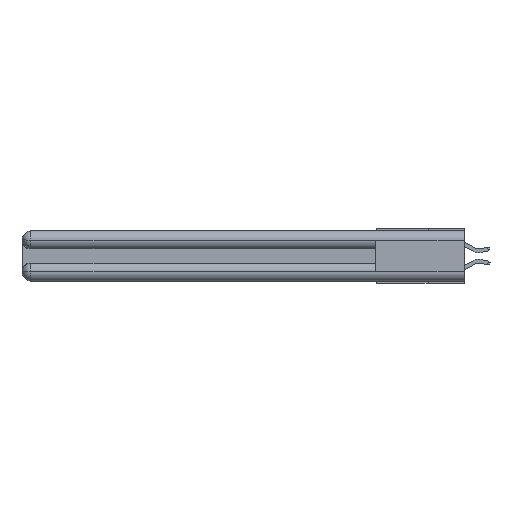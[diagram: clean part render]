
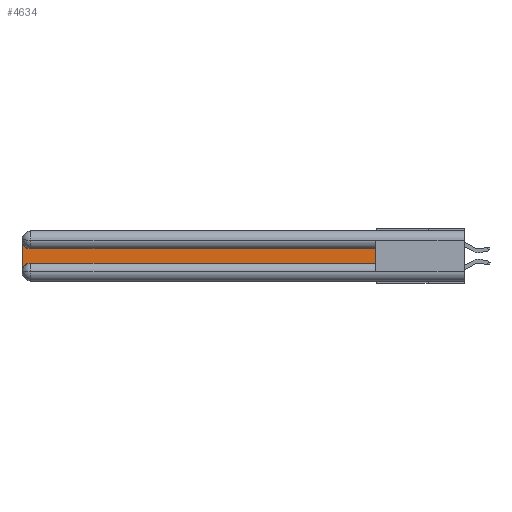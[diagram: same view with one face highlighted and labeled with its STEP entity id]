
A CAD part, left-side view. The second image highlights one B-rep face of the part: STEP entity #4634.
In plain terms, the highlighted planar face has unit normal (-1, 0, 0).
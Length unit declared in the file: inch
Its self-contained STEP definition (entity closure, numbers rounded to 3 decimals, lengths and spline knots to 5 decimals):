
#515 = VERTEX_POINT ( 'NONE', #25482 ) ;
#589 = CARTESIAN_POINT ( 'NONE',  ( 0.075, 2.94, -0.0625 ) ) ;
#709 = DIRECTION ( 'NONE',  ( 0., 0., -1. ) ) ;
#936 = DIRECTION ( 'NONE',  ( 1., 0., 0. ) ) ;
#1106 = LINE ( 'NONE', #28609, #12428 ) ;
#1406 = EDGE_CURVE ( 'NONE', #9785, #18341, #14608, .T. ) ;
#1716 = LINE ( 'NONE', #6207, #13897 ) ;
#3504 = CARTESIAN_POINT ( 'NONE',  ( 0.075, 3., -0.1225 ) ) ;
#4245 = VECTOR ( 'NONE', #32320, 39.37008 ) ;
#4634 = ADVANCED_FACE ( 'NONE', ( #17571 ), #8517, .F. ) ;
#5281 = CARTESIAN_POINT ( 'NONE',  ( 0.075, 2.94, -0.2775 ) ) ;
#5322 = EDGE_CURVE ( 'NONE', #18341, #7015, #23565, .T. ) ;
#6207 = CARTESIAN_POINT ( 'NONE',  ( 0.075, 0.6, -0.2175 ) ) ;
#7015 = VERTEX_POINT ( 'NONE', #17842 ) ;
#7834 = EDGE_CURVE ( 'NONE', #515, #26210, #1716, .T. ) ;
#8028 = LINE ( 'NONE', #23870, #4245 ) ;
#8517 = PLANE ( 'NONE',  #11452 ) ;
#9201 = CARTESIAN_POINT ( 'NONE',  ( 0.075, 0.6, -0.2175 ) ) ;
#9785 = VERTEX_POINT ( 'NONE', #31864 ) ;
#10254 = ORIENTED_EDGE ( 'NONE', *, *, #11381, .T. ) ;
#10398 = DIRECTION ( 'NONE',  ( 0., 0., -1. ) ) ;
#11381 = EDGE_CURVE ( 'NONE', #7015, #515, #17368, .T. ) ;
#11452 = AXIS2_PLACEMENT_3D ( 'NONE', #3504, #936, #27818 ) ;
#11609 = AXIS2_PLACEMENT_3D ( 'NONE', #589, #32872, #709 ) ;
#12428 = VECTOR ( 'NONE', #12513, 39.37008 ) ;
#12513 = DIRECTION ( 'NONE',  ( 0., 0., 1. ) ) ;
#13598 = ORIENTED_EDGE ( 'NONE', *, *, #15460, .T. ) ;
#13897 = VECTOR ( 'NONE', #33085, 39.37008 ) ;
#14351 = AXIS2_PLACEMENT_3D ( 'NONE', #5281, #26530, #10398 ) ;
#14608 = CIRCLE ( 'NONE', #11609, 0.06 ) ;
#14615 = DIRECTION ( 'NONE',  ( 0., 0., -1. ) ) ;
#15460 = EDGE_CURVE ( 'NONE', #26210, #25555, #1106, .T. ) ;
#17368 = CIRCLE ( 'NONE', #14351, 0.06 ) ;
#17571 = FACE_OUTER_BOUND ( 'NONE', #31752, .T. ) ;
#17842 = CARTESIAN_POINT ( 'NONE',  ( 0.075, 3., -0.2775 ) ) ;
#18116 = ORIENTED_EDGE ( 'NONE', *, *, #1406, .T. ) ;
#18341 = VERTEX_POINT ( 'NONE', #26505 ) ;
#19365 = ORIENTED_EDGE ( 'NONE', *, *, #7834, .T. ) ;
#19434 = ORIENTED_EDGE ( 'NONE', *, *, #28910, .T. ) ;
#23565 = LINE ( 'NONE', #25300, #32817 ) ;
#23870 = CARTESIAN_POINT ( 'NONE',  ( 0.075, 0.6, -0.1225 ) ) ;
#25300 = CARTESIAN_POINT ( 'NONE',  ( 0.075, 3., -0.2175 ) ) ;
#25482 = CARTESIAN_POINT ( 'NONE',  ( 0.075, 2.94, -0.2175 ) ) ;
#25555 = VERTEX_POINT ( 'NONE', #33470 ) ;
#26210 = VERTEX_POINT ( 'NONE', #9201 ) ;
#26505 = CARTESIAN_POINT ( 'NONE',  ( 0.075, 3., -0.0625 ) ) ;
#26530 = DIRECTION ( 'NONE',  ( 1., 0., 0. ) ) ;
#27818 = DIRECTION ( 'NONE',  ( 0., 0., -1. ) ) ;
#28609 = CARTESIAN_POINT ( 'NONE',  ( 0.075, 0.6, -0.2175 ) ) ;
#28910 = EDGE_CURVE ( 'NONE', #25555, #9785, #8028, .T. ) ;
#30645 = ORIENTED_EDGE ( 'NONE', *, *, #5322, .T. ) ;
#31752 = EDGE_LOOP ( 'NONE', ( #19434, #18116, #30645, #10254, #19365, #13598 ) ) ;
#31864 = CARTESIAN_POINT ( 'NONE',  ( 0.075, 2.94, -0.1225 ) ) ;
#32320 = DIRECTION ( 'NONE',  ( 0., 1., 0. ) ) ;
#32817 = VECTOR ( 'NONE', #14615, 39.37008 ) ;
#32872 = DIRECTION ( 'NONE',  ( 1., 0., 0. ) ) ;
#33085 = DIRECTION ( 'NONE',  ( 0., -1., 0. ) ) ;
#33470 = CARTESIAN_POINT ( 'NONE',  ( 0.075, 0.6, -0.1225 ) ) ;
